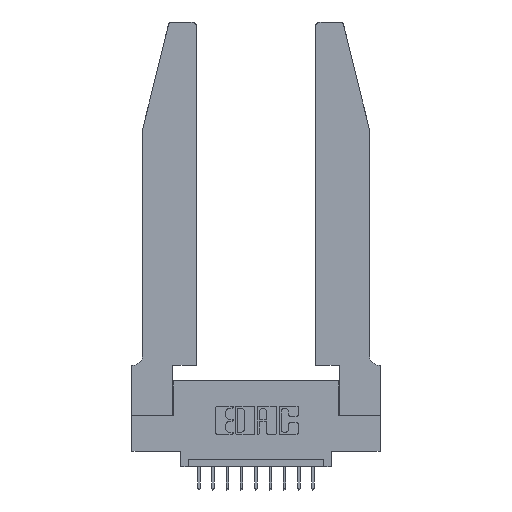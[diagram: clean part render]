
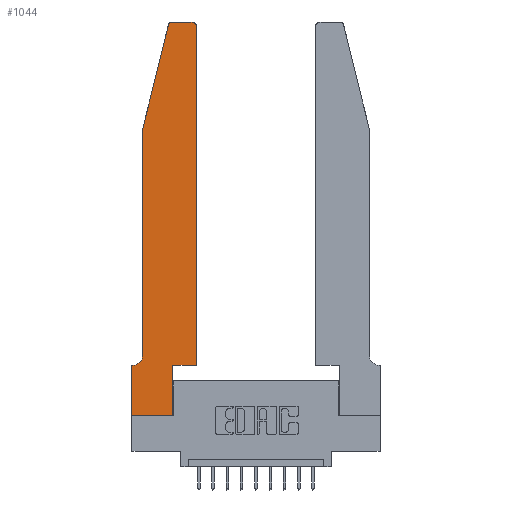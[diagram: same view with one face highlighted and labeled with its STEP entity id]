
A CAD part, top view. The second image highlights one B-rep face of the part: STEP entity #1044.
In plain terms, the highlighted planar face has unit normal (0, 0, 1).
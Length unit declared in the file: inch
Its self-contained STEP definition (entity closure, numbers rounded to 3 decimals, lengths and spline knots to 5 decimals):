
#56 = LINE ( 'NONE', #14648, #13736 ) ;
#81 = CARTESIAN_POINT ( 'NONE',  ( 0.0755, 2., 0.37 ) ) ;
#97 = ORIENTED_EDGE ( 'NONE', *, *, #1742, .T. ) ;
#406 = LINE ( 'NONE', #14290, #11956 ) ;
#588 = LINE ( 'NONE', #16061, #2716 ) ;
#719 = CARTESIAN_POINT ( 'NONE',  ( 0.4505, 2.72, 0.37 ) ) ;
#845 = EDGE_CURVE ( 'NONE', #2268, #11380, #9608, .T. ) ;
#1044 = ADVANCED_FACE ( 'NONE', ( #11164 ), #15009, .T. ) ;
#1179 = VERTEX_POINT ( 'NONE', #14144 ) ;
#1285 = DIRECTION ( 'NONE',  ( 0., -1., 0. ) ) ;
#1408 = DIRECTION ( 'NONE',  ( 1., 0., 0. ) ) ;
#1699 = LINE ( 'NONE', #13691, #14405 ) ;
#1719 = CARTESIAN_POINT ( 'NONE',  ( 0., 0., 0.37 ) ) ;
#1742 = EDGE_CURVE ( 'NONE', #11440, #9937, #16010, .T. ) ;
#2071 = DIRECTION ( 'NONE',  ( -1., 0., 0. ) ) ;
#2268 = VERTEX_POINT ( 'NONE', #5434 ) ;
#2271 = CARTESIAN_POINT ( 'NONE',  ( 0.284, 2.75, 0.37 ) ) ;
#2339 = EDGE_CURVE ( 'NONE', #4879, #5664, #4165, .T. ) ;
#2565 = ORIENTED_EDGE ( 'NONE', *, *, #10767, .T. ) ;
#2716 = VECTOR ( 'NONE', #7257, 39.37008 ) ;
#2794 = CIRCLE ( 'NONE', #11356, 0.03 ) ;
#3481 = VECTOR ( 'NONE', #16111, 39.37008 ) ;
#3571 = VERTEX_POINT ( 'NONE', #7886 ) ;
#3575 = ORIENTED_EDGE ( 'NONE', *, *, #9913, .T. ) ;
#3717 = AXIS2_PLACEMENT_3D ( 'NONE', #15819, #10877, #12264 ) ;
#4165 = LINE ( 'NONE', #1719, #4473 ) ;
#4260 = DIRECTION ( 'NONE',  ( 1., 0., 0. ) ) ;
#4291 = EDGE_CURVE ( 'NONE', #15886, #11440, #2794, .T. ) ;
#4470 = DIRECTION ( 'NONE',  ( 1., 0., 0. ) ) ;
#4473 = VECTOR ( 'NONE', #11732, 39.37008 ) ;
#4497 = CARTESIAN_POINT ( 'NONE',  ( 0.0055, 0.42, 0.37 ) ) ;
#4849 = VECTOR ( 'NONE', #1285, 39.37008 ) ;
#4879 = VERTEX_POINT ( 'NONE', #14434 ) ;
#5026 = EDGE_CURVE ( 'NONE', #11380, #4879, #5846, .T. ) ;
#5424 = DIRECTION ( 'NONE',  ( 1., 0., 0. ) ) ;
#5434 = CARTESIAN_POINT ( 'NONE',  ( 0.0755, 0.42, 0.37 ) ) ;
#5556 = ORIENTED_EDGE ( 'NONE', *, *, #12894, .T. ) ;
#5664 = VERTEX_POINT ( 'NONE', #9916 ) ;
#5704 = VERTEX_POINT ( 'NONE', #11340 ) ;
#5846 = LINE ( 'NONE', #13057, #12161 ) ;
#6211 = ORIENTED_EDGE ( 'NONE', *, *, #2339, .T. ) ;
#6398 = CARTESIAN_POINT ( 'NONE',  ( 0.2865, 0.35, 0.37 ) ) ;
#6511 = EDGE_CURVE ( 'NONE', #5664, #1179, #406, .T. ) ;
#6659 = CARTESIAN_POINT ( 'NONE',  ( 0.0055, 0.35, 0.37 ) ) ;
#6664 = CARTESIAN_POINT ( 'NONE',  ( 0.4205, 2.72, 0.37 ) ) ;
#7241 = AXIS2_PLACEMENT_3D ( 'NONE', #12564, #11199, #1408 ) ;
#7257 = DIRECTION ( 'NONE',  ( 0., 1., 0. ) ) ;
#7289 = DIRECTION ( 'NONE',  ( -0.239, -0.971, 0. ) ) ;
#7459 = AXIS2_PLACEMENT_3D ( 'NONE', #4497, #8305, #2071 ) ;
#7788 = CARTESIAN_POINT ( 'NONE',  ( 0.25487, 2.72718, 0.37 ) ) ;
#7886 = CARTESIAN_POINT ( 'NONE',  ( 0.4505, 0.35, 0.37 ) ) ;
#7986 = DIRECTION ( 'NONE',  ( -1., 0., 0. ) ) ;
#8305 = DIRECTION ( 'NONE',  ( 0., 0., -1. ) ) ;
#8556 = ORIENTED_EDGE ( 'NONE', *, *, #12362, .T. ) ;
#8782 = EDGE_CURVE ( 'NONE', #14197, #5704, #1699, .T. ) ;
#9305 = CARTESIAN_POINT ( 'NONE',  ( 0.4205, 2.75, 0.37 ) ) ;
#9378 = LINE ( 'NONE', #9843, #3481 ) ;
#9489 = ORIENTED_EDGE ( 'NONE', *, *, #5026, .T. ) ;
#9608 = CIRCLE ( 'NONE', #7459, 0.07 ) ;
#9843 = CARTESIAN_POINT ( 'NONE',  ( 0.4505, 0.35, 0.37 ) ) ;
#9913 = EDGE_CURVE ( 'NONE', #9937, #14197, #14748, .T. ) ;
#9916 = CARTESIAN_POINT ( 'NONE',  ( 0., 0., 0.37 ) ) ;
#9937 = VERTEX_POINT ( 'NONE', #2271 ) ;
#10127 = DIRECTION ( 'NONE',  ( -1., 0., 0. ) ) ;
#10351 = VECTOR ( 'NONE', #10127, 39.37008 ) ;
#10406 = DIRECTION ( 'NONE',  ( 0., 0., 1. ) ) ;
#10767 = EDGE_CURVE ( 'NONE', #16186, #3571, #56, .T. ) ;
#10877 = DIRECTION ( 'NONE',  ( 0., 0., 1. ) ) ;
#11164 = FACE_OUTER_BOUND ( 'NONE', #13910, .T. ) ;
#11199 = DIRECTION ( 'NONE',  ( 0., 0., 1. ) ) ;
#11243 = ORIENTED_EDGE ( 'NONE', *, *, #8782, .T. ) ;
#11339 = CARTESIAN_POINT ( 'NONE',  ( 0.2605, 2.75, 0.37 ) ) ;
#11340 = CARTESIAN_POINT ( 'NONE',  ( 0.0755, 2., 0.37 ) ) ;
#11356 = AXIS2_PLACEMENT_3D ( 'NONE', #6664, #10406, #5424 ) ;
#11380 = VERTEX_POINT ( 'NONE', #6659 ) ;
#11440 = VERTEX_POINT ( 'NONE', #9305 ) ;
#11732 = DIRECTION ( 'NONE',  ( 0., -1., 0. ) ) ;
#11956 = VECTOR ( 'NONE', #4260, 39.37008 ) ;
#12161 = VECTOR ( 'NONE', #7986, 39.37008 ) ;
#12193 = ORIENTED_EDGE ( 'NONE', *, *, #6511, .T. ) ;
#12244 = ORIENTED_EDGE ( 'NONE', *, *, #4291, .T. ) ;
#12264 = DIRECTION ( 'NONE',  ( 1., 0., 0. ) ) ;
#12362 = EDGE_CURVE ( 'NONE', #5704, #2268, #13304, .T. ) ;
#12564 = CARTESIAN_POINT ( 'NONE',  ( 0., 0.35, 0.37 ) ) ;
#12889 = EDGE_CURVE ( 'NONE', #3571, #15886, #9378, .T. ) ;
#12894 = EDGE_CURVE ( 'NONE', #1179, #16186, #588, .T. ) ;
#13057 = CARTESIAN_POINT ( 'NONE',  ( 0.0755, 0.35, 0.37 ) ) ;
#13304 = LINE ( 'NONE', #81, #4849 ) ;
#13425 = ORIENTED_EDGE ( 'NONE', *, *, #12889, .T. ) ;
#13691 = CARTESIAN_POINT ( 'NONE',  ( 0.0755, 2., 0.37 ) ) ;
#13736 = VECTOR ( 'NONE', #4470, 39.37008 ) ;
#13910 = EDGE_LOOP ( 'NONE', ( #97, #3575, #11243, #8556, #15054, #9489, #6211, #12193, #5556, #2565, #13425, #12244 ) ) ;
#14144 = CARTESIAN_POINT ( 'NONE',  ( 0.2865, 0., 0.37 ) ) ;
#14197 = VERTEX_POINT ( 'NONE', #7788 ) ;
#14290 = CARTESIAN_POINT ( 'NONE',  ( 0., 0., 0.37 ) ) ;
#14405 = VECTOR ( 'NONE', #7289, 39.37008 ) ;
#14434 = CARTESIAN_POINT ( 'NONE',  ( 0., 0.35, 0.37 ) ) ;
#14648 = CARTESIAN_POINT ( 'NONE',  ( 0.4505, 0.35, 0.37 ) ) ;
#14748 = CIRCLE ( 'NONE', #3717, 0.03 ) ;
#15009 = PLANE ( 'NONE',  #7241 ) ;
#15054 = ORIENTED_EDGE ( 'NONE', *, *, #845, .T. ) ;
#15819 = CARTESIAN_POINT ( 'NONE',  ( 0.284, 2.72, 0.37 ) ) ;
#15886 = VERTEX_POINT ( 'NONE', #719 ) ;
#16010 = LINE ( 'NONE', #11339, #10351 ) ;
#16061 = CARTESIAN_POINT ( 'NONE',  ( 0.2865, 0.35, 0.37 ) ) ;
#16111 = DIRECTION ( 'NONE',  ( 0., 1., 0. ) ) ;
#16186 = VERTEX_POINT ( 'NONE', #6398 ) ;
